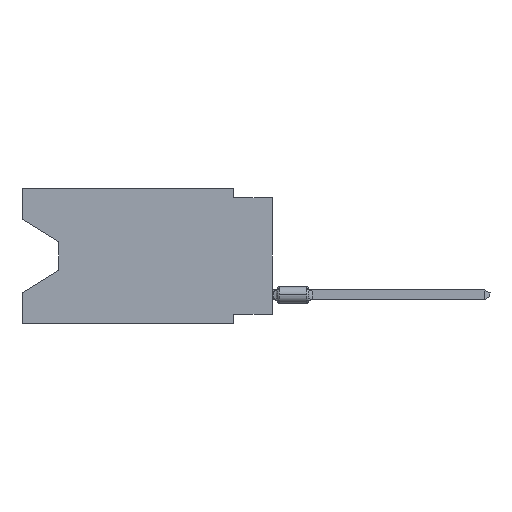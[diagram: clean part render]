
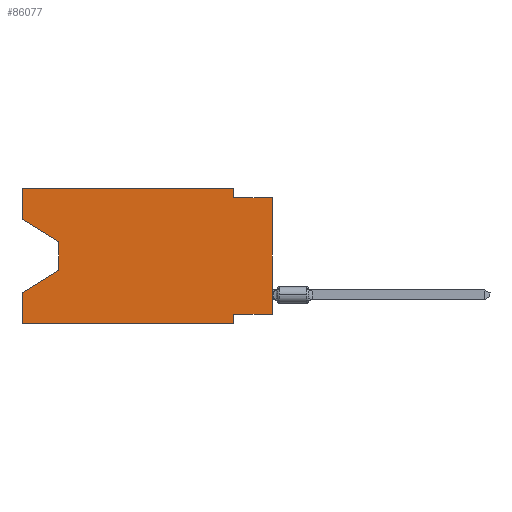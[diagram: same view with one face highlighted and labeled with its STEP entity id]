
A CAD part, left-side view. The second image highlights one B-rep face of the part: STEP entity #86077.
In plain terms, the highlighted planar face has unit normal (-1, 0, 0).
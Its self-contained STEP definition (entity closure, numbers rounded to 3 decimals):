
#278 = EDGE_CURVE ( 'NONE', #90547, #69671, #95580, .T. ) ;
#475 = CARTESIAN_POINT ( 'NONE',  ( 0., 16.383, -8.89 ) ) ;
#640 = EDGE_CURVE ( 'NONE', #96659, #38831, #53324, .T. ) ;
#1627 = ORIENTED_EDGE ( 'NONE', *, *, #99373, .F. ) ;
#1927 = CARTESIAN_POINT ( 'NONE',  ( 0., 16.383, 0. ) ) ;
#2013 = CARTESIAN_POINT ( 'NONE',  ( 0., 0., 0. ) ) ;
#3793 = DIRECTION ( 'NONE',  ( 0., -1., 0. ) ) ;
#6035 = ORIENTED_EDGE ( 'NONE', *, *, #278, .T. ) ;
#6166 = EDGE_CURVE ( 'NONE', #33106, #69263, #24649, .T. ) ;
#10475 = CARTESIAN_POINT ( 'NONE',  ( 0., 16.383, -6.852 ) ) ;
#10907 = CARTESIAN_POINT ( 'NONE',  ( 0., 0., -0.635 ) ) ;
#12194 = VECTOR ( 'NONE', #66298, 1000. ) ;
#14874 = CARTESIAN_POINT ( 'NONE',  ( 0., 2.54, -8.89 ) ) ;
#15377 = AXIS2_PLACEMENT_3D ( 'NONE', #83450, #74490, #26008 ) ;
#16972 = CARTESIAN_POINT ( 'NONE',  ( 0., 0., -8.255 ) ) ;
#17210 = ORIENTED_EDGE ( 'NONE', *, *, #66911, .T. ) ;
#18564 = EDGE_CURVE ( 'NONE', #49352, #23913, #26731, .T. ) ;
#23261 = CARTESIAN_POINT ( 'NONE',  ( 0., 0., -8.255 ) ) ;
#23659 = VECTOR ( 'NONE', #46993, 1000. ) ;
#23913 = VERTEX_POINT ( 'NONE', #91664 ) ;
#24649 = LINE ( 'NONE', #1927, #90211 ) ;
#26008 = DIRECTION ( 'NONE',  ( 0., 0., -1. ) ) ;
#26731 = LINE ( 'NONE', #10907, #96733 ) ;
#26928 = CARTESIAN_POINT ( 'NONE',  ( 0., 2.54, 0. ) ) ;
#28831 = CARTESIAN_POINT ( 'NONE',  ( 0., 13.97, -3.505 ) ) ;
#29624 = VERTEX_POINT ( 'NONE', #32085 ) ;
#32085 = CARTESIAN_POINT ( 'NONE',  ( 0., 16.383, -2.038 ) ) ;
#32941 = DIRECTION ( 'NONE',  ( 0., 0., -1. ) ) ;
#33106 = VERTEX_POINT ( 'NONE', #75106 ) ;
#34119 = CARTESIAN_POINT ( 'NONE',  ( 0., 2.54, -8.255 ) ) ;
#35348 = ORIENTED_EDGE ( 'NONE', *, *, #58159, .T. ) ;
#36624 = VERTEX_POINT ( 'NONE', #26928 ) ;
#37030 = CARTESIAN_POINT ( 'NONE',  ( 0., 13.97, -5.385 ) ) ;
#37143 = VECTOR ( 'NONE', #60974, 1000. ) ;
#38157 = CARTESIAN_POINT ( 'NONE',  ( 0., 16.383, 0. ) ) ;
#38168 = CARTESIAN_POINT ( 'NONE',  ( 0., 13.97, -5.385 ) ) ;
#38249 = DIRECTION ( 'NONE',  ( 0., 0., 1. ) ) ;
#38831 = VERTEX_POINT ( 'NONE', #34119 ) ;
#40298 = VECTOR ( 'NONE', #51756, 1000. ) ;
#40548 = LINE ( 'NONE', #475, #77741 ) ;
#40975 = DIRECTION ( 'NONE',  ( 0., 0., 1. ) ) ;
#43513 = ORIENTED_EDGE ( 'NONE', *, *, #18564, .F. ) ;
#44490 = ORIENTED_EDGE ( 'NONE', *, *, #50839, .F. ) ;
#44742 = CARTESIAN_POINT ( 'NONE',  ( 0., 2.54, 0. ) ) ;
#45508 = ORIENTED_EDGE ( 'NONE', *, *, #640, .F. ) ;
#46993 = DIRECTION ( 'NONE',  ( 0., 1., 0. ) ) ;
#48780 = EDGE_CURVE ( 'NONE', #69671, #69263, #54994, .T. ) ;
#49352 = VERTEX_POINT ( 'NONE', #64316 ) ;
#50401 = VECTOR ( 'NONE', #93490, 1000. ) ;
#50839 = EDGE_CURVE ( 'NONE', #73838, #36624, #75989, .T. ) ;
#51193 = VECTOR ( 'NONE', #3793, 1000. ) ;
#51756 = DIRECTION ( 'NONE',  ( 0., -0.855, -0.519 ) ) ;
#53324 = LINE ( 'NONE', #23261, #23659 ) ;
#54029 = ORIENTED_EDGE ( 'NONE', *, *, #89288, .T. ) ;
#54257 = ORIENTED_EDGE ( 'NONE', *, *, #48780, .T. ) ;
#54548 = CARTESIAN_POINT ( 'NONE',  ( 0., 16.383, 0. ) ) ;
#54994 = LINE ( 'NONE', #38168, #50401 ) ;
#56383 = VECTOR ( 'NONE', #32941, 1000. ) ;
#57677 = LINE ( 'NONE', #98235, #56383 ) ;
#58088 = LINE ( 'NONE', #91811, #40298 ) ;
#58159 = EDGE_CURVE ( 'NONE', #29624, #90547, #58088, .T. ) ;
#58660 = ORIENTED_EDGE ( 'NONE', *, *, #82827, .F. ) ;
#59868 = ORIENTED_EDGE ( 'NONE', *, *, #68671, .F. ) ;
#60974 = DIRECTION ( 'NONE',  ( 0., 0., -1. ) ) ;
#64316 = CARTESIAN_POINT ( 'NONE',  ( 0., 2.54, -0.635 ) ) ;
#66298 = DIRECTION ( 'NONE',  ( 0., 0., 1. ) ) ;
#66911 = EDGE_CURVE ( 'NONE', #33106, #93924, #40548, .T. ) ;
#66987 = CARTESIAN_POINT ( 'NONE',  ( 0., 13.97, -3.505 ) ) ;
#67095 = PLANE ( 'NONE',  #15377 ) ;
#68671 = EDGE_CURVE ( 'NONE', #29624, #73838, #79305, .T. ) ;
#69263 = VERTEX_POINT ( 'NONE', #10475 ) ;
#69671 = VERTEX_POINT ( 'NONE', #37030 ) ;
#72252 = VECTOR ( 'NONE', #76860, 1000. ) ;
#73838 = VERTEX_POINT ( 'NONE', #38157 ) ;
#74222 = LINE ( 'NONE', #2013, #12194 ) ;
#74490 = DIRECTION ( 'NONE',  ( 1., 0., 0. ) ) ;
#75106 = CARTESIAN_POINT ( 'NONE',  ( 0., 16.383, -8.89 ) ) ;
#75989 = LINE ( 'NONE', #76501, #51193 ) ;
#76501 = CARTESIAN_POINT ( 'NONE',  ( 0., 16.383, 0. ) ) ;
#76860 = DIRECTION ( 'NONE',  ( 0., 0., -1. ) ) ;
#77459 = EDGE_LOOP ( 'NONE', ( #35348, #6035, #54257, #102037, #17210, #1627, #45508, #54029, #43513, #58660, #44490, #59868 ) ) ;
#77741 = VECTOR ( 'NONE', #84739, 1000. ) ;
#79305 = LINE ( 'NONE', #54548, #85013 ) ;
#82827 = EDGE_CURVE ( 'NONE', #36624, #49352, #92679, .T. ) ;
#83450 = CARTESIAN_POINT ( 'NONE',  ( 0., 16.383, 0. ) ) ;
#84739 = DIRECTION ( 'NONE',  ( 0., -1., 0. ) ) ;
#85013 = VECTOR ( 'NONE', #38249, 1000. ) ;
#86077 = ADVANCED_FACE ( 'NONE', ( #98201 ), #67095, .F. ) ;
#89288 = EDGE_CURVE ( 'NONE', #96659, #23913, #74222, .T. ) ;
#89984 = DIRECTION ( 'NONE',  ( 0., -1., 0. ) ) ;
#90211 = VECTOR ( 'NONE', #40975, 1000. ) ;
#90547 = VERTEX_POINT ( 'NONE', #66987 ) ;
#91664 = CARTESIAN_POINT ( 'NONE',  ( 0., 0., -0.635 ) ) ;
#91811 = CARTESIAN_POINT ( 'NONE',  ( 0., 16.383, -2.038 ) ) ;
#92679 = LINE ( 'NONE', #44742, #72252 ) ;
#93490 = DIRECTION ( 'NONE',  ( 0., 0.855, -0.519 ) ) ;
#93924 = VERTEX_POINT ( 'NONE', #14874 ) ;
#95580 = LINE ( 'NONE', #28831, #37143 ) ;
#96659 = VERTEX_POINT ( 'NONE', #16972 ) ;
#96733 = VECTOR ( 'NONE', #89984, 1000. ) ;
#98201 = FACE_OUTER_BOUND ( 'NONE', #77459, .T. ) ;
#98235 = CARTESIAN_POINT ( 'NONE',  ( 0., 2.54, -8.89 ) ) ;
#99373 = EDGE_CURVE ( 'NONE', #38831, #93924, #57677, .T. ) ;
#102037 = ORIENTED_EDGE ( 'NONE', *, *, #6166, .F. ) ;
